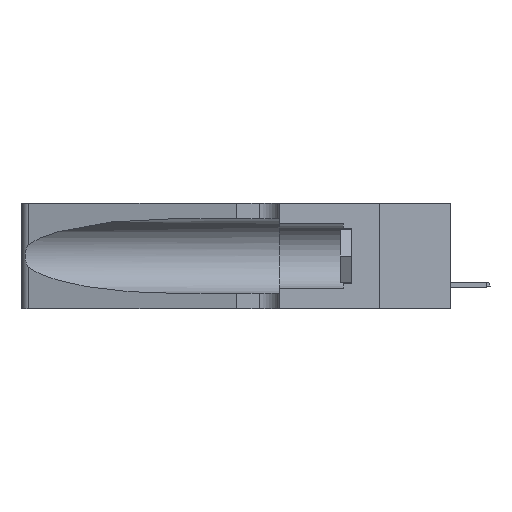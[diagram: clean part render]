
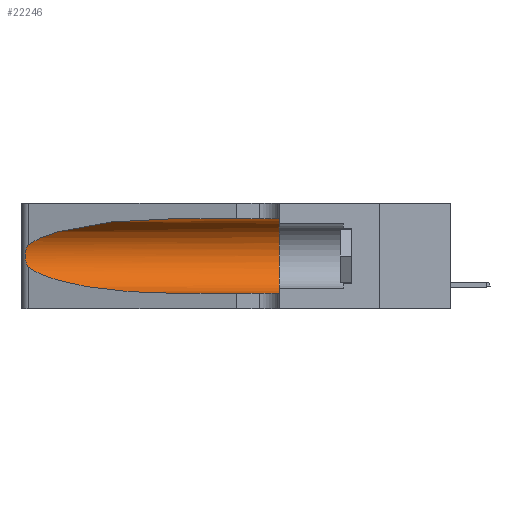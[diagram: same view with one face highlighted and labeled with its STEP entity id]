
A CAD part, left-side view. The second image highlights one B-rep face of the part: STEP entity #22246.
In plain terms, the highlighted cylindrical face has radius 3.308 mm (diameter 6.617 mm), a partial arc.
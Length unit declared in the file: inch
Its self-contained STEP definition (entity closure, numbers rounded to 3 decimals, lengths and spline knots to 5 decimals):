
#216 =( BOUNDED_CURVE ( )  B_SPLINE_CURVE ( 3, ( #16972, #23251, #21530, #14810 ),
 .UNSPECIFIED., .F., .T. ) 
 B_SPLINE_CURVE_WITH_KNOTS ( ( 4, 4 ),
 ( 1.5708, 2.84003 ),
 .UNSPECIFIED. ) 
 CURVE ( )  GEOMETRIC_REPRESENTATION_ITEM ( )  RATIONAL_B_SPLINE_CURVE ( ( 1., 0.87, 0.87, 1. ) ) 
 REPRESENTATION_ITEM ( '' )  );
#755 = CARTESIAN_POINT ( 'NONE',  ( 0.25555, 1.22994, 0.2215 ) ) ;
#900 = CARTESIAN_POINT ( 'NONE',  ( 0.25639, 1.23186, 0.15144 ) ) ;
#2152 = CARTESIAN_POINT ( 'NONE',  ( 0.1305, 1.61858, 0.31525 ) ) ;
#2197 = EDGE_LOOP ( 'NONE', ( #21708, #6553, #17390, #23085, #18091, #4645 ) ) ;
#2530 = CARTESIAN_POINT ( 'NONE',  ( 0.1305, 1.61858, 0.185 ) ) ;
#3048 = CARTESIAN_POINT ( 'NONE',  ( 0.26018, 1.23835, 0.19895 ) ) ;
#3333 = CARTESIAN_POINT ( 'NONE',  ( 0.25639, 1.23184, 0.21858 ) ) ;
#4645 = ORIENTED_EDGE ( 'NONE', *, *, #11313, .F. ) ;
#4907 = CARTESIAN_POINT ( 'NONE',  ( 0.25555, 1.22993, 0.14849 ) ) ;
#5233 = VERTEX_POINT ( 'NONE', #20843 ) ;
#5324 = VERTEX_POINT ( 'NONE', #20276 ) ;
#5333 = CARTESIAN_POINT ( 'NONE',  ( 0.25856, 1.23593, 0.16098 ) ) ;
#5715 = CIRCLE ( 'NONE', #27179, 0.13025 ) ;
#6553 = ORIENTED_EDGE ( 'NONE', *, *, #24830, .T. ) ;
#6813 = VECTOR ( 'NONE', #24166, 39.37008 ) ;
#7052 = CARTESIAN_POINT ( 'NONE',  ( 0.1305, 0.35, 0.185 ) ) ;
#7396 = DIRECTION ( 'NONE',  ( 0., -1., 0. ) ) ;
#8314 = CARTESIAN_POINT ( 'NONE',  ( 0.1305, 0.35, 0.05475 ) ) ;
#9474 = CARTESIAN_POINT ( 'NONE',  ( 0.26075, 1.23896, 0.19203 ) ) ;
#9646 = CARTESIAN_POINT ( 'NONE',  ( 0.1305, 0.72297, 0.05475 ) ) ;
#10059 = VECTOR ( 'NONE', #7396, 39.37008 ) ;
#10444 = CARTESIAN_POINT ( 'NONE',  ( 0.1305, 0.72297, 0.05475 ) ) ;
#10822 = CYLINDRICAL_SURFACE ( 'NONE', #14439, 0.13025 ) ;
#11242 = DIRECTION ( 'NONE',  ( 0., -1., 0. ) ) ;
#11313 = EDGE_CURVE ( 'NONE', #20751, #14987, #19878, .T. ) ;
#11741 =( BOUNDED_CURVE ( )  B_SPLINE_CURVE ( 3, ( #16901, #12597, #21322, #10444 ),
 .UNSPECIFIED., .F., .F. ) 
 B_SPLINE_CURVE_WITH_KNOTS ( ( 4, 4 ),
 ( 3.44316, 4.71239 ),
 .UNSPECIFIED. ) 
 CURVE ( )  GEOMETRIC_REPRESENTATION_ITEM ( )  RATIONAL_B_SPLINE_CURVE ( ( 1., 0.87, 0.87, 1. ) ) 
 REPRESENTATION_ITEM ( '' )  );
#11762 = CARTESIAN_POINT ( 'NONE',  ( 0.25487, 1.22718, 0.14631 ) ) ;
#12597 = CARTESIAN_POINT ( 'NONE',  ( 0.2373, 1.15595, 0.08982 ) ) ;
#13247 = B_SPLINE_CURVE_WITH_KNOTS ( 'NONE', 3,
 ( #24494, #755, #3333, #20355, #15780, #3048, #9474, #24636, #13785, #5333, #22641, #900, #4907, #11762 ),
 .UNSPECIFIED., .F., .F.,
 ( 4, 2, 2, 2, 2, 2, 4 ),
 ( 0., 0.00027, 0.00053, 0.00107, 0.0016, 0.00187, 0.00214 ),
 .UNSPECIFIED. ) ;
#13785 = CARTESIAN_POINT ( 'NONE',  ( 0.26017, 1.23833, 0.17102 ) ) ;
#14123 = CARTESIAN_POINT ( 'NONE',  ( 0.1305, 0.35, 0.31525 ) ) ;
#14439 = AXIS2_PLACEMENT_3D ( 'NONE', #2530, #11242, #19707 ) ;
#14726 = EDGE_CURVE ( 'NONE', #24052, #20184, #27145, .T. ) ;
#14810 = CARTESIAN_POINT ( 'NONE',  ( 0.25487, 1.22718, 0.22369 ) ) ;
#14987 = VERTEX_POINT ( 'NONE', #14123 ) ;
#15780 = CARTESIAN_POINT ( 'NONE',  ( 0.25854, 1.2359, 0.20912 ) ) ;
#16901 = CARTESIAN_POINT ( 'NONE',  ( 0.25487, 1.22718, 0.14631 ) ) ;
#16972 = CARTESIAN_POINT ( 'NONE',  ( 0.1305, 0.72297, 0.31525 ) ) ;
#17390 = ORIENTED_EDGE ( 'NONE', *, *, #28098, .T. ) ;
#18078 = DIRECTION ( 'NONE',  ( 0., 1., 0. ) ) ;
#18091 = ORIENTED_EDGE ( 'NONE', *, *, #24822, .F. ) ;
#19707 = DIRECTION ( 'NONE',  ( 0., 0., -1. ) ) ;
#19837 = FACE_OUTER_BOUND ( 'NONE', #2197, .T. ) ;
#19878 = LINE ( 'NONE', #2152, #6813 ) ;
#20184 = VERTEX_POINT ( 'NONE', #8314 ) ;
#20276 = CARTESIAN_POINT ( 'NONE',  ( 0.25487, 1.22718, 0.14631 ) ) ;
#20355 = CARTESIAN_POINT ( 'NONE',  ( 0.25787, 1.23484, 0.2124 ) ) ;
#20426 = CARTESIAN_POINT ( 'NONE',  ( 0.1305, 0.72297, 0.31525 ) ) ;
#20751 = VERTEX_POINT ( 'NONE', #20426 ) ;
#20843 = CARTESIAN_POINT ( 'NONE',  ( 0.25487, 1.22718, 0.22369 ) ) ;
#21322 = CARTESIAN_POINT ( 'NONE',  ( 0.18966, 0.96281, 0.05475 ) ) ;
#21530 = CARTESIAN_POINT ( 'NONE',  ( 0.2373, 1.15595, 0.28018 ) ) ;
#21708 = ORIENTED_EDGE ( 'NONE', *, *, #25883, .T. ) ;
#22246 = ADVANCED_FACE ( 'NONE', ( #19837 ), #10822, .F. ) ;
#22641 = CARTESIAN_POINT ( 'NONE',  ( 0.25789, 1.23486, 0.15765 ) ) ;
#23085 = ORIENTED_EDGE ( 'NONE', *, *, #14726, .T. ) ;
#23251 = CARTESIAN_POINT ( 'NONE',  ( 0.18966, 0.96281, 0.31525 ) ) ;
#24052 = VERTEX_POINT ( 'NONE', #9646 ) ;
#24166 = DIRECTION ( 'NONE',  ( 0., -1., 0. ) ) ;
#24494 = CARTESIAN_POINT ( 'NONE',  ( 0.25487, 1.22718, 0.22369 ) ) ;
#24636 = CARTESIAN_POINT ( 'NONE',  ( 0.26075, 1.23896, 0.178 ) ) ;
#24822 = EDGE_CURVE ( 'NONE', #14987, #20184, #5715, .T. ) ;
#24830 = EDGE_CURVE ( 'NONE', #5233, #5324, #13247, .T. ) ;
#25883 = EDGE_CURVE ( 'NONE', #20751, #5233, #216, .T. ) ;
#26796 = DIRECTION ( 'NONE',  ( 0., 0., 1. ) ) ;
#26856 = CARTESIAN_POINT ( 'NONE',  ( 0.1305, 1.61858, 0.05475 ) ) ;
#27145 = LINE ( 'NONE', #26856, #10059 ) ;
#27179 = AXIS2_PLACEMENT_3D ( 'NONE', #7052, #18078, #26796 ) ;
#28098 = EDGE_CURVE ( 'NONE', #5324, #24052, #11741, .T. ) ;
